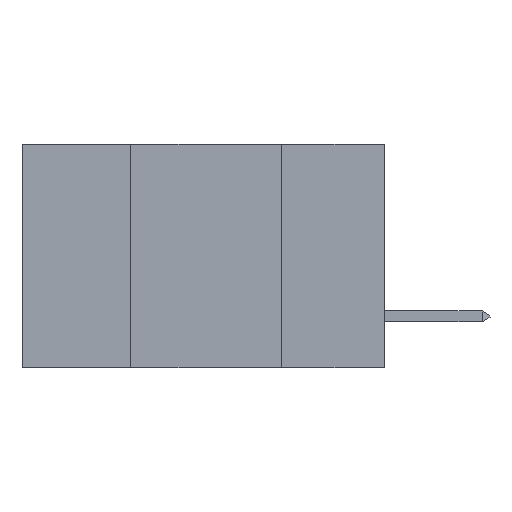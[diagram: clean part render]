
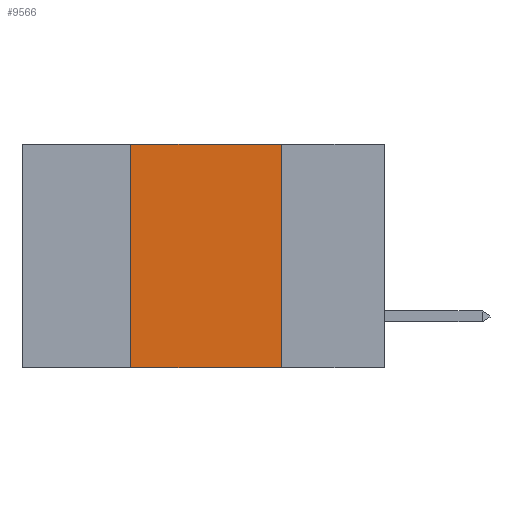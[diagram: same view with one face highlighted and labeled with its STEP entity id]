
A CAD part, left-side view. The second image highlights one B-rep face of the part: STEP entity #9566.
In plain terms, the highlighted planar face has unit normal (-1, 0, 0).
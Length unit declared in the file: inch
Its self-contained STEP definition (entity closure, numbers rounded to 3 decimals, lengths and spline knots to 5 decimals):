
#90 = DIRECTION ( 'NONE',  ( 0., -1., 0. ) ) ;
#424 = CARTESIAN_POINT ( 'NONE',  ( 0., 0.17, 0. ) ) ;
#1208 = ORIENTED_EDGE ( 'NONE', *, *, #13105, .F. ) ;
#1685 = DIRECTION ( 'NONE',  ( 0., 0., -1. ) ) ;
#1728 = CARTESIAN_POINT ( 'NONE',  ( 0., 0.17, -0.37 ) ) ;
#1752 = CARTESIAN_POINT ( 'NONE',  ( 0., 0.42, -0.37 ) ) ;
#2307 = VERTEX_POINT ( 'NONE', #10579 ) ;
#2351 = VECTOR ( 'NONE', #13857, 39.37008 ) ;
#2740 = ORIENTED_EDGE ( 'NONE', *, *, #8884, .T. ) ;
#4621 = ORIENTED_EDGE ( 'NONE', *, *, #8770, .F. ) ;
#5276 = LINE ( 'NONE', #6970, #10676 ) ;
#5718 = VERTEX_POINT ( 'NONE', #1752 ) ;
#6148 = EDGE_CURVE ( 'NONE', #6774, #9165, #7393, .T. ) ;
#6262 = DIRECTION ( 'NONE',  ( 0., 0., -1. ) ) ;
#6774 = VERTEX_POINT ( 'NONE', #424 ) ;
#6970 = CARTESIAN_POINT ( 'NONE',  ( 0., 0.6, 0. ) ) ;
#6998 = EDGE_LOOP ( 'NONE', ( #7568, #4621, #1208, #2740 ) ) ;
#7393 = LINE ( 'NONE', #18292, #18211 ) ;
#7568 = ORIENTED_EDGE ( 'NONE', *, *, #6148, .F. ) ;
#8528 = DIRECTION ( 'NONE',  ( 0., -1., 0. ) ) ;
#8770 = EDGE_CURVE ( 'NONE', #2307, #6774, #5276, .T. ) ;
#8884 = EDGE_CURVE ( 'NONE', #5718, #9165, #15139, .T. ) ;
#9118 = CARTESIAN_POINT ( 'NONE',  ( 0., 0.6, -0.37 ) ) ;
#9165 = VERTEX_POINT ( 'NONE', #1728 ) ;
#9566 = ADVANCED_FACE ( 'NONE', ( #12047 ), #18236, .F. ) ;
#10579 = CARTESIAN_POINT ( 'NONE',  ( 0., 0.42, 0. ) ) ;
#10676 = VECTOR ( 'NONE', #8528, 39.37008 ) ;
#12047 = FACE_OUTER_BOUND ( 'NONE', #6998, .T. ) ;
#13105 = EDGE_CURVE ( 'NONE', #5718, #2307, #15542, .T. ) ;
#13857 = DIRECTION ( 'NONE',  ( 0., 0., 1. ) ) ;
#15040 = CARTESIAN_POINT ( 'NONE',  ( 0., 0.6, 0. ) ) ;
#15139 = LINE ( 'NONE', #9118, #16800 ) ;
#15255 = DIRECTION ( 'NONE',  ( 1., 0., 0. ) ) ;
#15542 = LINE ( 'NONE', #16924, #2351 ) ;
#16800 = VECTOR ( 'NONE', #90, 39.37008 ) ;
#16924 = CARTESIAN_POINT ( 'NONE',  ( 0., 0.42, 0. ) ) ;
#17248 = AXIS2_PLACEMENT_3D ( 'NONE', #15040, #15255, #1685 ) ;
#18211 = VECTOR ( 'NONE', #6262, 39.37008 ) ;
#18236 = PLANE ( 'NONE',  #17248 ) ;
#18292 = CARTESIAN_POINT ( 'NONE',  ( 0., 0.17, 0. ) ) ;
